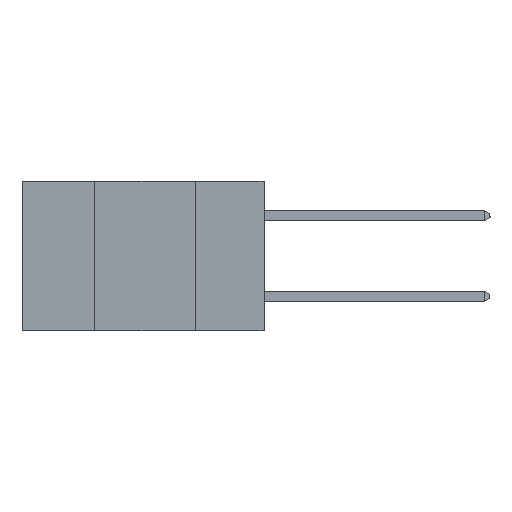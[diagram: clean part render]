
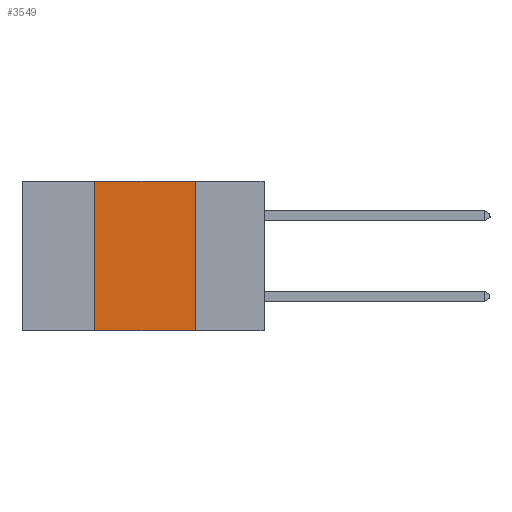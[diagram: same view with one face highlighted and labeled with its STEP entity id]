
A CAD part, left-side view. The second image highlights one B-rep face of the part: STEP entity #3549.
In plain terms, the highlighted planar face has unit normal (-1, 0, 0).
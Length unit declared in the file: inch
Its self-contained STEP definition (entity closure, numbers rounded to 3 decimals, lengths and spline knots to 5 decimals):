
#2523 = EDGE_CURVE ( 'NONE', #10602, #23870, #4893, .T. ) ;
#3549 = ADVANCED_FACE ( 'NONE', ( #9933 ), #5660, .F. ) ;
#3867 = EDGE_CURVE ( 'NONE', #10602, #9908, #17828, .T. ) ;
#4559 = VECTOR ( 'NONE', #15695, 39.37008 ) ;
#4893 = LINE ( 'NONE', #13555, #14416 ) ;
#5065 = VERTEX_POINT ( 'NONE', #18368 ) ;
#5660 = PLANE ( 'NONE',  #21358 ) ;
#6345 = DIRECTION ( 'NONE',  ( 0., 0., -1. ) ) ;
#6478 = DIRECTION ( 'NONE',  ( 1., 0., 0. ) ) ;
#6520 = CARTESIAN_POINT ( 'NONE',  ( 0., 0.6, 0. ) ) ;
#7194 = DIRECTION ( 'NONE',  ( 0., 0., -1. ) ) ;
#8289 = ORIENTED_EDGE ( 'NONE', *, *, #2523, .T. ) ;
#8908 = ORIENTED_EDGE ( 'NONE', *, *, #3867, .F. ) ;
#9319 = EDGE_CURVE ( 'NONE', #5065, #23870, #10680, .T. ) ;
#9908 = VERTEX_POINT ( 'NONE', #25594 ) ;
#9933 = FACE_OUTER_BOUND ( 'NONE', #15290, .T. ) ;
#10602 = VERTEX_POINT ( 'NONE', #17396 ) ;
#10680 = LINE ( 'NONE', #19327, #20831 ) ;
#10826 = DIRECTION ( 'NONE',  ( 0., 0., 1. ) ) ;
#12420 = ORIENTED_EDGE ( 'NONE', *, *, #9319, .F. ) ;
#13555 = CARTESIAN_POINT ( 'NONE',  ( 0., 0.6, -0.37 ) ) ;
#14416 = VECTOR ( 'NONE', #24875, 39.37008 ) ;
#15290 = EDGE_LOOP ( 'NONE', ( #12420, #25723, #8908, #8289 ) ) ;
#15695 = DIRECTION ( 'NONE',  ( 0., -1., 0. ) ) ;
#17174 = CARTESIAN_POINT ( 'NONE',  ( 0., 0.17, -0.37 ) ) ;
#17396 = CARTESIAN_POINT ( 'NONE',  ( 0., 0.42, -0.37 ) ) ;
#17828 = LINE ( 'NONE', #21294, #22587 ) ;
#18368 = CARTESIAN_POINT ( 'NONE',  ( 0., 0.17, 0. ) ) ;
#19327 = CARTESIAN_POINT ( 'NONE',  ( 0., 0.17, 0. ) ) ;
#20760 = LINE ( 'NONE', #25797, #4559 ) ;
#20831 = VECTOR ( 'NONE', #7194, 39.37008 ) ;
#21294 = CARTESIAN_POINT ( 'NONE',  ( 0., 0.42, 0. ) ) ;
#21358 = AXIS2_PLACEMENT_3D ( 'NONE', #6520, #6478, #6345 ) ;
#22587 = VECTOR ( 'NONE', #10826, 39.37008 ) ;
#23870 = VERTEX_POINT ( 'NONE', #17174 ) ;
#23914 = EDGE_CURVE ( 'NONE', #9908, #5065, #20760, .T. ) ;
#24875 = DIRECTION ( 'NONE',  ( 0., -1., 0. ) ) ;
#25594 = CARTESIAN_POINT ( 'NONE',  ( 0., 0.42, 0. ) ) ;
#25723 = ORIENTED_EDGE ( 'NONE', *, *, #23914, .F. ) ;
#25797 = CARTESIAN_POINT ( 'NONE',  ( 0., 0.6, 0. ) ) ;
